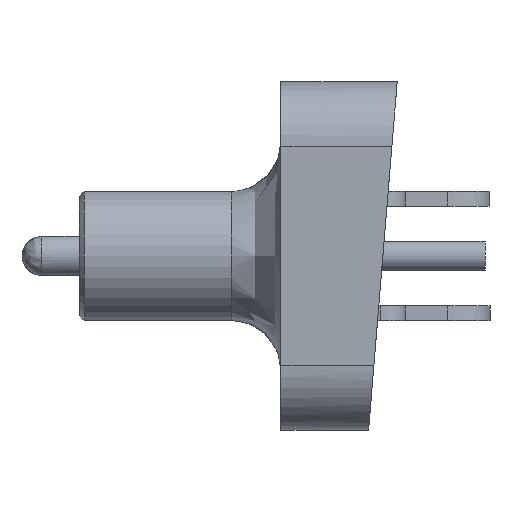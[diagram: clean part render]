
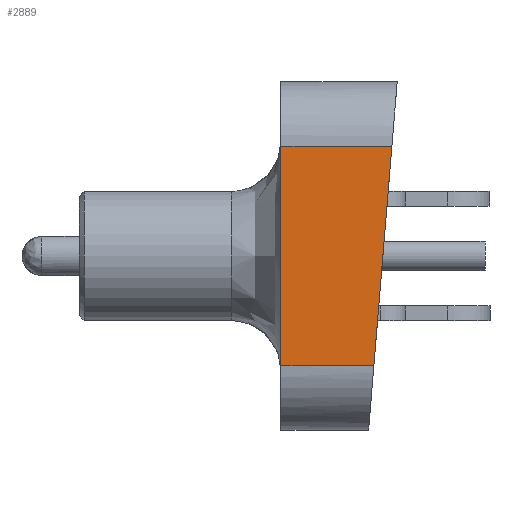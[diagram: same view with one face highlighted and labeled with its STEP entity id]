
A CAD part, left-side view. The second image highlights one B-rep face of the part: STEP entity #2889.
In plain terms, the highlighted planar face has unit normal (-1, 0, 0).
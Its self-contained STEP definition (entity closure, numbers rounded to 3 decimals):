
#331 = VERTEX_POINT ( 'NONE', #14309 ) ;
#380 = CARTESIAN_POINT ( 'NONE',  ( -24.637, 12.13, -2.82 ) ) ;
#1452 = CARTESIAN_POINT ( 'NONE',  ( -24.637, 11.015, -0.62 ) ) ;
#1982 = EDGE_CURVE ( 'NONE', #331, #3660, #8283, .T. ) ;
#2889 = ADVANCED_FACE ( 'NONE', ( #15263 ), #13174, .T. ) ;
#3660 = VERTEX_POINT ( 'NONE', #6767 ) ;
#3708 = ORIENTED_EDGE ( 'NONE', *, *, #1982, .T. ) ;
#3892 = VECTOR ( 'NONE', #4609, 1000. ) ;
#3982 = VECTOR ( 'NONE', #14122, 1000. ) ;
#4289 = DIRECTION ( 'NONE',  ( -1., 0., 0. ) ) ;
#4609 = DIRECTION ( 'NONE',  ( 0., -0.082, 0.997 ) ) ;
#4873 = EDGE_CURVE ( 'NONE', #3660, #13223, #10732, .T. ) ;
#5100 = CARTESIAN_POINT ( 'NONE',  ( -24.637, 13.296, -0.62 ) ) ;
#5630 = LINE ( 'NONE', #15677, #13377 ) ;
#6495 = ORIENTED_EDGE ( 'NONE', *, *, #14267, .T. ) ;
#6767 = CARTESIAN_POINT ( 'NONE',  ( -24.637, 11.377, -5.02 ) ) ;
#8283 = LINE ( 'NONE', #14769, #12145 ) ;
#9094 = LINE ( 'NONE', #5100, #3982 ) ;
#9110 = DIRECTION ( 'NONE',  ( 0., 0., -1. ) ) ;
#9557 = DIRECTION ( 'NONE',  ( 0., 0., 1. ) ) ;
#10732 = LINE ( 'NONE', #13427, #3892 ) ;
#11739 = CARTESIAN_POINT ( 'NONE',  ( -24.637, 13.244, -0.62 ) ) ;
#12145 = VECTOR ( 'NONE', #13426, 1000. ) ;
#12384 = ORIENTED_EDGE ( 'NONE', *, *, #16273, .F. ) ;
#13174 = PLANE ( 'NONE',  #13810 ) ;
#13223 = VERTEX_POINT ( 'NONE', #1452 ) ;
#13377 = VECTOR ( 'NONE', #9110, 1000. ) ;
#13426 = DIRECTION ( 'NONE',  ( 0., -1., 0. ) ) ;
#13427 = CARTESIAN_POINT ( 'NONE',  ( -24.637, 11.196, -2.82 ) ) ;
#13810 = AXIS2_PLACEMENT_3D ( 'NONE', #380, #4289, #9557 ) ;
#14122 = DIRECTION ( 'NONE',  ( 0., -1., 0. ) ) ;
#14267 = EDGE_CURVE ( 'NONE', #14776, #331, #5630, .T. ) ;
#14304 = ORIENTED_EDGE ( 'NONE', *, *, #4873, .T. ) ;
#14309 = CARTESIAN_POINT ( 'NONE',  ( -24.637, 13.244, -5.02 ) ) ;
#14477 = EDGE_LOOP ( 'NONE', ( #6495, #3708, #14304, #12384 ) ) ;
#14769 = CARTESIAN_POINT ( 'NONE',  ( -24.637, 12.13, -5.02 ) ) ;
#14776 = VERTEX_POINT ( 'NONE', #11739 ) ;
#15263 = FACE_OUTER_BOUND ( 'NONE', #14477, .T. ) ;
#15677 = CARTESIAN_POINT ( 'NONE',  ( -24.637, 13.244, -2.82 ) ) ;
#16273 = EDGE_CURVE ( 'NONE', #14776, #13223, #9094, .T. ) ;
